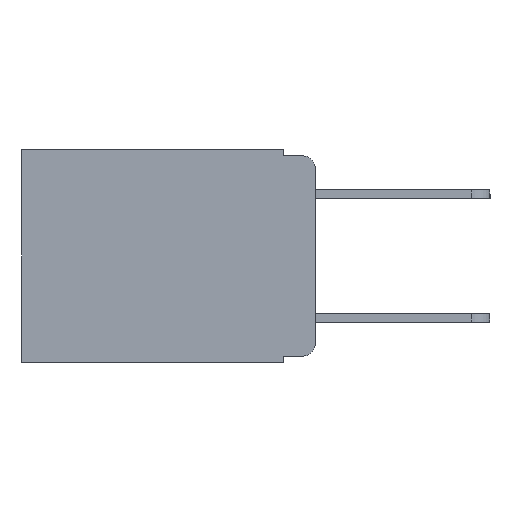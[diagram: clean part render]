
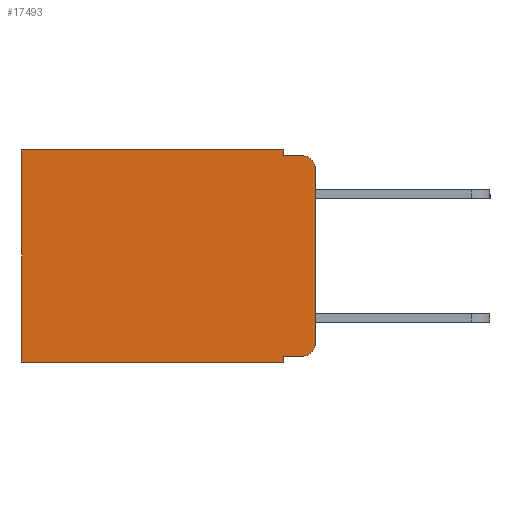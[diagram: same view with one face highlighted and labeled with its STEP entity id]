
A CAD part, left-side view. The second image highlights one B-rep face of the part: STEP entity #17493.
In plain terms, the highlighted planar face has unit normal (-1, 0, 0).
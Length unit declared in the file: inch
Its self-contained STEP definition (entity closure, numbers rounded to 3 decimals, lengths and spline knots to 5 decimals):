
#23 = EDGE_CURVE ( 'NONE', #363, #8348, #18378, .T. ) ;
#151 = LINE ( 'NONE', #18440, #10173 ) ;
#363 = VERTEX_POINT ( 'NONE', #2506 ) ;
#498 = LINE ( 'NONE', #5800, #10505 ) ;
#676 = EDGE_CURVE ( 'NONE', #24196, #1992, #4706, .T. ) ;
#1212 = LINE ( 'NONE', #6035, #21311 ) ;
#1341 = DIRECTION ( 'NONE',  ( 0., 0., -1. ) ) ;
#1412 = VERTEX_POINT ( 'NONE', #14265 ) ;
#1992 = VERTEX_POINT ( 'NONE', #21951 ) ;
#2239 = VECTOR ( 'NONE', #17072, 39.37008 ) ;
#2431 = CARTESIAN_POINT ( 'NONE',  ( 0.298, 0.051, 0. ) ) ;
#2506 = CARTESIAN_POINT ( 'NONE',  ( 0.298, 0.02, -0.333 ) ) ;
#2577 = DIRECTION ( 'NONE',  ( 0., 0., -1. ) ) ;
#2954 = EDGE_CURVE ( 'NONE', #22454, #6340, #498, .T. ) ;
#4452 = DIRECTION ( 'NONE',  ( 0., 0., -1. ) ) ;
#4581 = ORIENTED_EDGE ( 'NONE', *, *, #676, .T. ) ;
#4706 = LINE ( 'NONE', #11118, #10613 ) ;
#5244 = ORIENTED_EDGE ( 'NONE', *, *, #17881, .T. ) ;
#5594 = EDGE_LOOP ( 'NONE', ( #6253, #12690, #9601, #13454, #4581, #5244, #11958, #9581, #21492, #8307 ) ) ;
#5800 = CARTESIAN_POINT ( 'NONE',  ( 0.298, 0., -0.343 ) ) ;
#6035 = CARTESIAN_POINT ( 'NONE',  ( 0.298, 0.051, -0.333 ) ) ;
#6253 = ORIENTED_EDGE ( 'NONE', *, *, #12326, .F. ) ;
#6320 = VERTEX_POINT ( 'NONE', #20450 ) ;
#6340 = VERTEX_POINT ( 'NONE', #12416 ) ;
#6757 = VERTEX_POINT ( 'NONE', #12977 ) ;
#6829 = VERTEX_POINT ( 'NONE', #18704 ) ;
#7009 = EDGE_CURVE ( 'NONE', #1412, #6757, #10496, .T. ) ;
#8105 = DIRECTION ( 'NONE',  ( -1., 0., 0. ) ) ;
#8307 = ORIENTED_EDGE ( 'NONE', *, *, #23, .T. ) ;
#8348 = VERTEX_POINT ( 'NONE', #13974 ) ;
#9328 = DIRECTION ( 'NONE',  ( 0., 1., 0. ) ) ;
#9581 = ORIENTED_EDGE ( 'NONE', *, *, #21855, .F. ) ;
#9601 = ORIENTED_EDGE ( 'NONE', *, *, #16034, .F. ) ;
#10173 = VECTOR ( 'NONE', #20354, 39.37008 ) ;
#10496 = CIRCLE ( 'NONE', #20829, 0.02 ) ;
#10505 = VECTOR ( 'NONE', #9328, 39.37008 ) ;
#10613 = VECTOR ( 'NONE', #11168, 39.37008 ) ;
#11118 = CARTESIAN_POINT ( 'NONE',  ( 0.298, 0., 0. ) ) ;
#11168 = DIRECTION ( 'NONE',  ( 0., 1., 0. ) ) ;
#11958 = ORIENTED_EDGE ( 'NONE', *, *, #2954, .F. ) ;
#12326 = EDGE_CURVE ( 'NONE', #1412, #8348, #14542, .T. ) ;
#12416 = CARTESIAN_POINT ( 'NONE',  ( 0.298, 0.473, -0.343 ) ) ;
#12690 = ORIENTED_EDGE ( 'NONE', *, *, #7009, .T. ) ;
#12721 = LINE ( 'NONE', #13190, #2239 ) ;
#12977 = CARTESIAN_POINT ( 'NONE',  ( 0.298, 0.02, -0.01 ) ) ;
#13142 = DIRECTION ( 'NONE',  ( 1., 0., 0. ) ) ;
#13190 = CARTESIAN_POINT ( 'NONE',  ( 0.298, 0.051, 0. ) ) ;
#13384 = DIRECTION ( 'NONE',  ( 0., 0., -1. ) ) ;
#13454 = ORIENTED_EDGE ( 'NONE', *, *, #19796, .F. ) ;
#13974 = CARTESIAN_POINT ( 'NONE',  ( 0.298, 0., -0.313 ) ) ;
#14238 = DIRECTION ( 'NONE',  ( -1., 0., 0. ) ) ;
#14265 = CARTESIAN_POINT ( 'NONE',  ( 0.298, 0., -0.03 ) ) ;
#14542 = LINE ( 'NONE', #24769, #16682 ) ;
#15620 = CARTESIAN_POINT ( 'NONE',  ( 0.298, 0.02, -0.313 ) ) ;
#15730 = DIRECTION ( 'NONE',  ( 0., -1., 0. ) ) ;
#15811 = DIRECTION ( 'NONE',  ( 0., 0., -1. ) ) ;
#15919 = CARTESIAN_POINT ( 'NONE',  ( 0.298, 0.051, -0.343 ) ) ;
#16034 = EDGE_CURVE ( 'NONE', #6320, #6757, #151, .T. ) ;
#16682 = VECTOR ( 'NONE', #13384, 39.37008 ) ;
#16686 = FACE_OUTER_BOUND ( 'NONE', #5594, .T. ) ;
#17072 = DIRECTION ( 'NONE',  ( 0., 0., -1. ) ) ;
#17493 = ADVANCED_FACE ( 'NONE', ( #16686 ), #20685, .F. ) ;
#17548 = VECTOR ( 'NONE', #2577, 39.37008 ) ;
#17770 = DIRECTION ( 'NONE',  ( 0., 0., -1. ) ) ;
#17881 = EDGE_CURVE ( 'NONE', #1992, #6340, #21987, .T. ) ;
#18049 = CARTESIAN_POINT ( 'NONE',  ( 0.298, 0.051, 0. ) ) ;
#18089 = CARTESIAN_POINT ( 'NONE',  ( 0.298, 0.473, 0. ) ) ;
#18378 = CIRCLE ( 'NONE', #20562, 0.02 ) ;
#18440 = CARTESIAN_POINT ( 'NONE',  ( 0.298, 0.051, -0.01 ) ) ;
#18704 = CARTESIAN_POINT ( 'NONE',  ( 0.298, 0.051, -0.333 ) ) ;
#18866 = CARTESIAN_POINT ( 'NONE',  ( 0.298, 0., 0. ) ) ;
#18944 = VECTOR ( 'NONE', #4452, 39.37008 ) ;
#19553 = LINE ( 'NONE', #18049, #18944 ) ;
#19672 = CARTESIAN_POINT ( 'NONE',  ( 0.298, 0.02, -0.03 ) ) ;
#19695 = EDGE_CURVE ( 'NONE', #6829, #363, #1212, .T. ) ;
#19796 = EDGE_CURVE ( 'NONE', #24196, #6320, #19553, .T. ) ;
#20354 = DIRECTION ( 'NONE',  ( 0., -1., 0. ) ) ;
#20450 = CARTESIAN_POINT ( 'NONE',  ( 0.298, 0.051, -0.01 ) ) ;
#20562 = AXIS2_PLACEMENT_3D ( 'NONE', #15620, #14238, #17770 ) ;
#20685 = PLANE ( 'NONE',  #21920 ) ;
#20829 = AXIS2_PLACEMENT_3D ( 'NONE', #19672, #8105, #15811 ) ;
#21311 = VECTOR ( 'NONE', #15730, 39.37008 ) ;
#21492 = ORIENTED_EDGE ( 'NONE', *, *, #19695, .T. ) ;
#21855 = EDGE_CURVE ( 'NONE', #6829, #22454, #12721, .T. ) ;
#21920 = AXIS2_PLACEMENT_3D ( 'NONE', #18866, #13142, #1341 ) ;
#21951 = CARTESIAN_POINT ( 'NONE',  ( 0.298, 0.473, 0. ) ) ;
#21987 = LINE ( 'NONE', #18089, #17548 ) ;
#22454 = VERTEX_POINT ( 'NONE', #15919 ) ;
#24196 = VERTEX_POINT ( 'NONE', #2431 ) ;
#24769 = CARTESIAN_POINT ( 'NONE',  ( 0.298, 0., 0. ) ) ;
